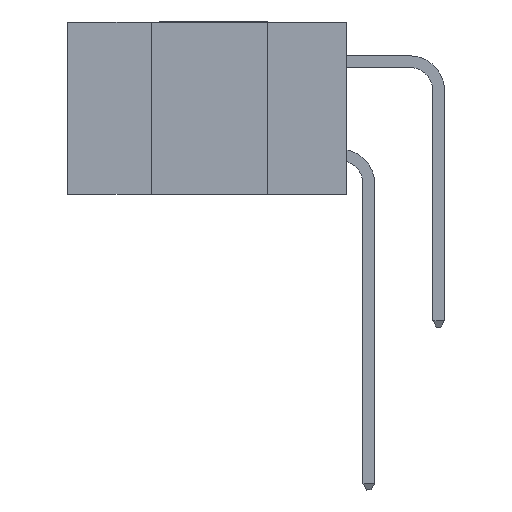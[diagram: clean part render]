
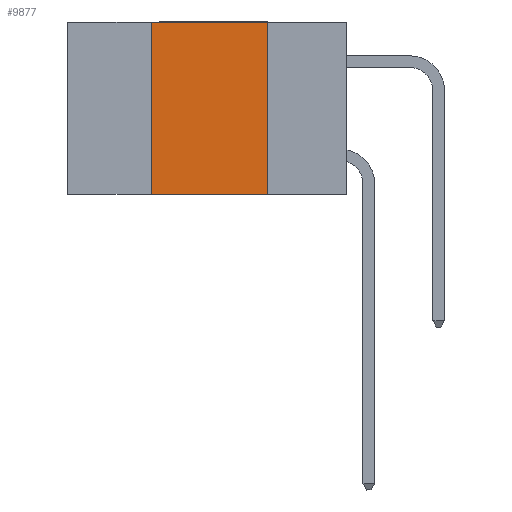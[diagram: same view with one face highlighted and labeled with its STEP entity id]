
A CAD part, left-side view. The second image highlights one B-rep face of the part: STEP entity #9877.
In plain terms, the highlighted planar face has unit normal (-1, 0, 0).
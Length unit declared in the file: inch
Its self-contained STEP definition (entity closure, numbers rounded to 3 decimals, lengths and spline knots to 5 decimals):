
#211 = ORIENTED_EDGE ( 'NONE', *, *, #1707, .F. ) ;
#368 = LINE ( 'NONE', #8072, #5180 ) ;
#1061 = VERTEX_POINT ( 'NONE', #6334 ) ;
#1084 = VECTOR ( 'NONE', #2653, 39.37008 ) ;
#1113 = CARTESIAN_POINT ( 'NONE',  ( 0., 0.42, 0. ) ) ;
#1119 = LINE ( 'NONE', #9652, #10348 ) ;
#1523 = DIRECTION ( 'NONE',  ( 0., -1., 0. ) ) ;
#1699 = EDGE_CURVE ( 'NONE', #3362, #1061, #10588, .T. ) ;
#1704 = ORIENTED_EDGE ( 'NONE', *, *, #4404, .T. ) ;
#1707 = EDGE_CURVE ( 'NONE', #9284, #4292, #10863, .T. ) ;
#2653 = DIRECTION ( 'NONE',  ( 0., 0., 1. ) ) ;
#2707 = CARTESIAN_POINT ( 'NONE',  ( 0., 0.17, 0. ) ) ;
#2710 = CARTESIAN_POINT ( 'NONE',  ( 0., 0.17, 0. ) ) ;
#3231 = DIRECTION ( 'NONE',  ( 0., -1., 0. ) ) ;
#3362 = VERTEX_POINT ( 'NONE', #2710 ) ;
#3690 = DIRECTION ( 'NONE',  ( 1., 0., 0. ) ) ;
#4225 = AXIS2_PLACEMENT_3D ( 'NONE', #10916, #3690, #10077 ) ;
#4292 = VERTEX_POINT ( 'NONE', #7060 ) ;
#4404 = EDGE_CURVE ( 'NONE', #9284, #1061, #368, .T. ) ;
#4515 = DIRECTION ( 'NONE',  ( 0., 0., -1. ) ) ;
#5180 = VECTOR ( 'NONE', #1523, 39.37008 ) ;
#5549 = EDGE_CURVE ( 'NONE', #4292, #3362, #1119, .T. ) ;
#6334 = CARTESIAN_POINT ( 'NONE',  ( 0., 0.17, -0.37 ) ) ;
#7060 = CARTESIAN_POINT ( 'NONE',  ( 0., 0.42, 0. ) ) ;
#7417 = PLANE ( 'NONE',  #4225 ) ;
#8072 = CARTESIAN_POINT ( 'NONE',  ( 0., 0.6, -0.37 ) ) ;
#8140 = FACE_OUTER_BOUND ( 'NONE', #11482, .T. ) ;
#8233 = VECTOR ( 'NONE', #4515, 39.37008 ) ;
#9262 = CARTESIAN_POINT ( 'NONE',  ( 0., 0.42, -0.37 ) ) ;
#9284 = VERTEX_POINT ( 'NONE', #9262 ) ;
#9652 = CARTESIAN_POINT ( 'NONE',  ( 0., 0.6, 0. ) ) ;
#9877 = ADVANCED_FACE ( 'NONE', ( #8140 ), #7417, .F. ) ;
#10077 = DIRECTION ( 'NONE',  ( 0., 0., -1. ) ) ;
#10348 = VECTOR ( 'NONE', #3231, 39.37008 ) ;
#10588 = LINE ( 'NONE', #2707, #8233 ) ;
#10863 = LINE ( 'NONE', #1113, #1084 ) ;
#10916 = CARTESIAN_POINT ( 'NONE',  ( 0., 0.6, 0. ) ) ;
#10960 = ORIENTED_EDGE ( 'NONE', *, *, #5549, .F. ) ;
#11362 = ORIENTED_EDGE ( 'NONE', *, *, #1699, .F. ) ;
#11482 = EDGE_LOOP ( 'NONE', ( #11362, #10960, #211, #1704 ) ) ;
